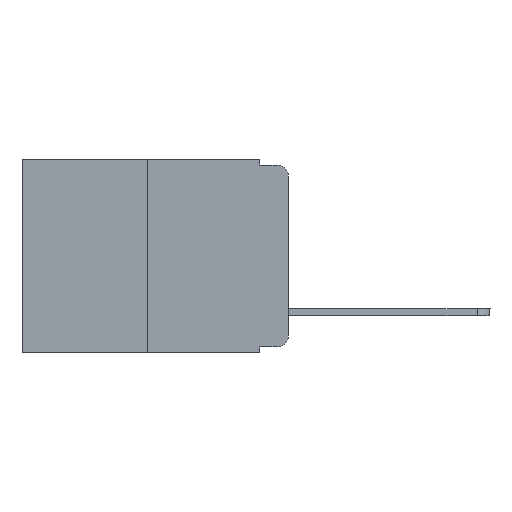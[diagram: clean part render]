
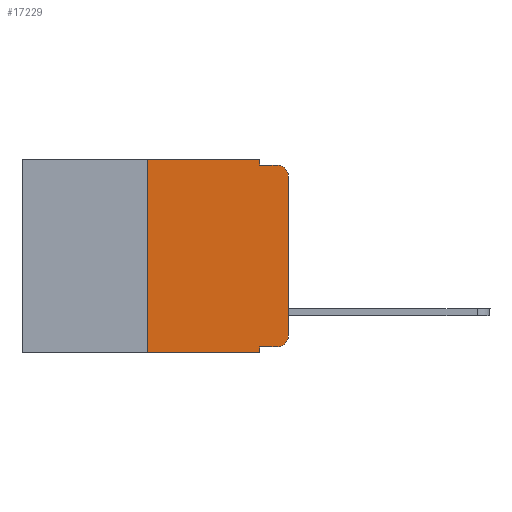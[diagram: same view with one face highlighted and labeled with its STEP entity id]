
A CAD part, left-side view. The second image highlights one B-rep face of the part: STEP entity #17229.
In plain terms, the highlighted planar face has unit normal (-1, 0, 0).
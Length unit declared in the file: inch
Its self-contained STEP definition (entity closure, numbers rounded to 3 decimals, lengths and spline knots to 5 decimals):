
#33 = CARTESIAN_POINT ( 'NONE',  ( 0., 0.25, 0. ) ) ;
#518 = EDGE_CURVE ( 'NONE', #20017, #11972, #20302, .T. ) ;
#661 = ORIENTED_EDGE ( 'NONE', *, *, #518, .F. ) ;
#812 = CARTESIAN_POINT ( 'NONE',  ( 0., 0.051, -0.01 ) ) ;
#1366 = VECTOR ( 'NONE', #8552, 39.37008 ) ;
#1639 = CARTESIAN_POINT ( 'NONE',  ( 0., 0.051, 0. ) ) ;
#1837 = CARTESIAN_POINT ( 'NONE',  ( 0., 0.25, 0. ) ) ;
#2502 = VECTOR ( 'NONE', #20889, 39.37008 ) ;
#2813 = DIRECTION ( 'NONE',  ( -1., 0., 0. ) ) ;
#2850 = FACE_OUTER_BOUND ( 'NONE', #4228, .T. ) ;
#3060 = CIRCLE ( 'NONE', #6453, 0.02 ) ;
#4222 = DIRECTION ( 'NONE',  ( 0., 0., 1. ) ) ;
#4228 = EDGE_LOOP ( 'NONE', ( #9852, #15160, #7812, #9557, #661, #12038, #4868, #8698, #16027, #6172 ) ) ;
#4807 = LINE ( 'NONE', #33, #12336 ) ;
#4868 = ORIENTED_EDGE ( 'NONE', *, *, #12821, .T. ) ;
#5354 = DIRECTION ( 'NONE',  ( 0., 0., -1. ) ) ;
#5577 = CARTESIAN_POINT ( 'NONE',  ( 0., 0.051, 0. ) ) ;
#5729 = DIRECTION ( 'NONE',  ( 0., -1., 0. ) ) ;
#5874 = EDGE_CURVE ( 'NONE', #11972, #13687, #17692, .T. ) ;
#6172 = ORIENTED_EDGE ( 'NONE', *, *, #9055, .T. ) ;
#6453 = AXIS2_PLACEMENT_3D ( 'NONE', #16401, #13214, #5354 ) ;
#6596 = EDGE_CURVE ( 'NONE', #6699, #18832, #13911, .T. ) ;
#6699 = VERTEX_POINT ( 'NONE', #8932 ) ;
#6934 = VECTOR ( 'NONE', #20117, 39.37008 ) ;
#7111 = CARTESIAN_POINT ( 'NONE',  ( 0., 0.02, -0.333 ) ) ;
#7217 = CARTESIAN_POINT ( 'NONE',  ( 0., 0., 0. ) ) ;
#7812 = ORIENTED_EDGE ( 'NONE', *, *, #16462, .F. ) ;
#8033 = EDGE_CURVE ( 'NONE', #11869, #10085, #3060, .T. ) ;
#8386 = CARTESIAN_POINT ( 'NONE',  ( 0., 0.02, -0.01 ) ) ;
#8552 = DIRECTION ( 'NONE',  ( 0., -1., 0. ) ) ;
#8698 = ORIENTED_EDGE ( 'NONE', *, *, #14127, .F. ) ;
#8763 = DIRECTION ( 'NONE',  ( 0., 0., -1. ) ) ;
#8932 = CARTESIAN_POINT ( 'NONE',  ( 0., 0.051, -0.333 ) ) ;
#8978 = CARTESIAN_POINT ( 'NONE',  ( 0., 0.02, -0.313 ) ) ;
#9055 = EDGE_CURVE ( 'NONE', #18832, #20301, #19269, .T. ) ;
#9557 = ORIENTED_EDGE ( 'NONE', *, *, #5874, .F. ) ;
#9561 = CARTESIAN_POINT ( 'NONE',  ( 0., 0., -0.03 ) ) ;
#9578 = VECTOR ( 'NONE', #4222, 39.37008 ) ;
#9852 = ORIENTED_EDGE ( 'NONE', *, *, #17067, .T. ) ;
#10085 = VERTEX_POINT ( 'NONE', #8386 ) ;
#10503 = CARTESIAN_POINT ( 'NONE',  ( 0., 0.051, 0. ) ) ;
#11031 = VERTEX_POINT ( 'NONE', #12117 ) ;
#11327 = VERTEX_POINT ( 'NONE', #18563 ) ;
#11869 = VERTEX_POINT ( 'NONE', #9561 ) ;
#11905 = CARTESIAN_POINT ( 'NONE',  ( 0., 0.473, 0. ) ) ;
#11953 = VECTOR ( 'NONE', #17368, 39.37008 ) ;
#11972 = VERTEX_POINT ( 'NONE', #10503 ) ;
#12038 = ORIENTED_EDGE ( 'NONE', *, *, #18191, .F. ) ;
#12117 = CARTESIAN_POINT ( 'NONE',  ( 0., 0.25, -0.343 ) ) ;
#12336 = VECTOR ( 'NONE', #19800, 39.37008 ) ;
#12719 = DIRECTION ( 'NONE',  ( 0., 0., -1. ) ) ;
#12821 = EDGE_CURVE ( 'NONE', #11031, #11327, #13333, .T. ) ;
#13214 = DIRECTION ( 'NONE',  ( -1., 0., 0. ) ) ;
#13333 = LINE ( 'NONE', #13534, #1366 ) ;
#13534 = CARTESIAN_POINT ( 'NONE',  ( 0., 0.473, -0.343 ) ) ;
#13687 = VERTEX_POINT ( 'NONE', #812 ) ;
#13686 = LINE ( 'NONE', #7217, #9578 ) ;
#13774 = VECTOR ( 'NONE', #8763, 39.37008 ) ;
#13911 = LINE ( 'NONE', #16699, #6934 ) ;
#14127 = EDGE_CURVE ( 'NONE', #6699, #11327, #16834, .T. ) ;
#14928 = VECTOR ( 'NONE', #5729, 39.37008 ) ;
#15160 = ORIENTED_EDGE ( 'NONE', *, *, #8033, .T. ) ;
#15673 = LINE ( 'NONE', #15881, #11953 ) ;
#15881 = CARTESIAN_POINT ( 'NONE',  ( 0., 0.051, -0.01 ) ) ;
#16027 = ORIENTED_EDGE ( 'NONE', *, *, #6596, .T. ) ;
#16226 = CARTESIAN_POINT ( 'NONE',  ( 0., 0.473, 0. ) ) ;
#16401 = CARTESIAN_POINT ( 'NONE',  ( 0., 0.02, -0.03 ) ) ;
#16462 = EDGE_CURVE ( 'NONE', #13687, #10085, #15673, .T. ) ;
#16699 = CARTESIAN_POINT ( 'NONE',  ( 0., 0.051, -0.333 ) ) ;
#16834 = LINE ( 'NONE', #5577, #13774 ) ;
#16884 = AXIS2_PLACEMENT_3D ( 'NONE', #8978, #2813, #17153 ) ;
#17067 = EDGE_CURVE ( 'NONE', #20301, #11869, #13686, .T. ) ;
#17153 = DIRECTION ( 'NONE',  ( 0., 0., -1. ) ) ;
#17229 = ADVANCED_FACE ( 'NONE', ( #2850 ), #20813, .F. ) ;
#17368 = DIRECTION ( 'NONE',  ( 0., -1., 0. ) ) ;
#17692 = LINE ( 'NONE', #1639, #2502 ) ;
#18191 = EDGE_CURVE ( 'NONE', #11031, #20017, #4807, .T. ) ;
#18563 = CARTESIAN_POINT ( 'NONE',  ( 0., 0.051, -0.343 ) ) ;
#18832 = VERTEX_POINT ( 'NONE', #7111 ) ;
#18923 = CARTESIAN_POINT ( 'NONE',  ( 0., 0., -0.313 ) ) ;
#19269 = CIRCLE ( 'NONE', #16884, 0.02 ) ;
#19313 = DIRECTION ( 'NONE',  ( 1., 0., 0. ) ) ;
#19800 = DIRECTION ( 'NONE',  ( 0., 0., 1. ) ) ;
#20017 = VERTEX_POINT ( 'NONE', #1837 ) ;
#20117 = DIRECTION ( 'NONE',  ( 0., -1., 0. ) ) ;
#20301 = VERTEX_POINT ( 'NONE', #18923 ) ;
#20302 = LINE ( 'NONE', #11905, #14928 ) ;
#20806 = AXIS2_PLACEMENT_3D ( 'NONE', #16226, #19313, #12719 ) ;
#20813 = PLANE ( 'NONE',  #20806 ) ;
#20889 = DIRECTION ( 'NONE',  ( 0., 0., -1. ) ) ;
